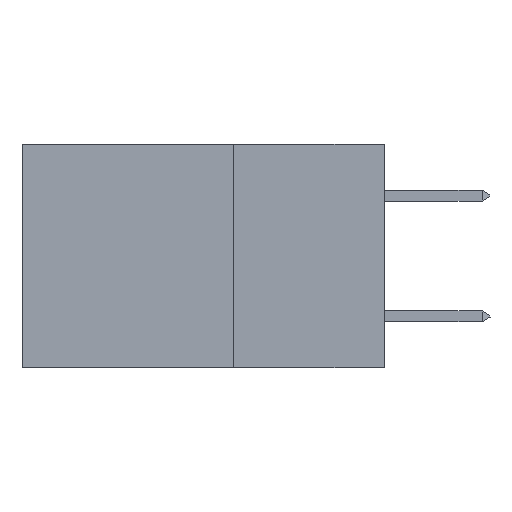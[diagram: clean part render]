
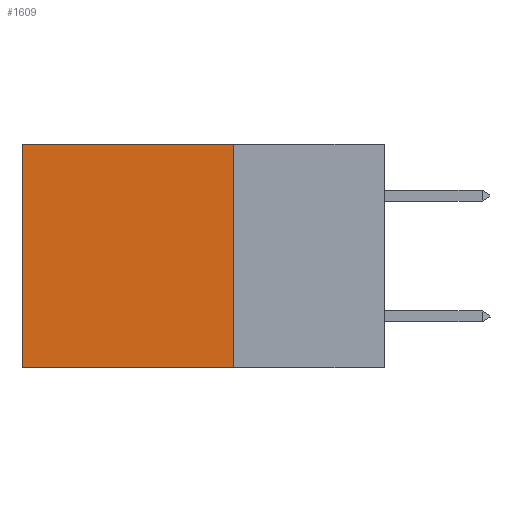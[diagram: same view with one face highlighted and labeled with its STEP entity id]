
A CAD part, left-side view. The second image highlights one B-rep face of the part: STEP entity #1609.
In plain terms, the highlighted planar face has unit normal (-1, 0, 0).
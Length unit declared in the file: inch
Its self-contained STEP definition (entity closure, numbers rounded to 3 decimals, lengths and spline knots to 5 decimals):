
#343 = CARTESIAN_POINT ( 'NONE',  ( 0.2875, 0.25, 0. ) ) ;
#895 = FACE_OUTER_BOUND ( 'NONE', #2288, .T. ) ;
#1002 = CARTESIAN_POINT ( 'NONE',  ( 0.2875, 0.25, -0.37 ) ) ;
#1474 = EDGE_CURVE ( 'NONE', #21234, #15775, #17273, .T. ) ;
#1609 = ADVANCED_FACE ( 'NONE', ( #895 ), #22056, .F. ) ;
#2288 = EDGE_LOOP ( 'NONE', ( #4274, #20066, #19866, #18275 ) ) ;
#3679 = LINE ( 'NONE', #343, #21585 ) ;
#4274 = ORIENTED_EDGE ( 'NONE', *, *, #13010, .T. ) ;
#5453 = CARTESIAN_POINT ( 'NONE',  ( 0.2875, 0.6, -0.37 ) ) ;
#7351 = CARTESIAN_POINT ( 'NONE',  ( 0.2875, 0.6, 0. ) ) ;
#7728 = LINE ( 'NONE', #12226, #21047 ) ;
#8316 = CARTESIAN_POINT ( 'NONE',  ( 0.2875, 0.25, 0. ) ) ;
#8322 = LINE ( 'NONE', #13500, #11852 ) ;
#10091 = DIRECTION ( 'NONE',  ( 0., 1., 0. ) ) ;
#10201 = DIRECTION ( 'NONE',  ( 0., 0., -1. ) ) ;
#10947 = DIRECTION ( 'NONE',  ( 0., 0., -1. ) ) ;
#11852 = VECTOR ( 'NONE', #10091, 39.37008 ) ;
#12226 = CARTESIAN_POINT ( 'NONE',  ( 0.2875, 0.6, 0. ) ) ;
#12547 = EDGE_CURVE ( 'NONE', #21234, #17060, #3679, .T. ) ;
#12642 = VECTOR ( 'NONE', #17256, 39.37008 ) ;
#13010 = EDGE_CURVE ( 'NONE', #15775, #17253, #7728, .T. ) ;
#13500 = CARTESIAN_POINT ( 'NONE',  ( 0.2875, 0.25, -0.37 ) ) ;
#13959 = DIRECTION ( 'NONE',  ( 0., 0., -1. ) ) ;
#15333 = DIRECTION ( 'NONE',  ( 1., 0., 0. ) ) ;
#15775 = VERTEX_POINT ( 'NONE', #7351 ) ;
#16700 = CARTESIAN_POINT ( 'NONE',  ( 0.2875, 0.25, 0. ) ) ;
#16953 = CARTESIAN_POINT ( 'NONE',  ( 0.2875, 0.25, 0. ) ) ;
#17060 = VERTEX_POINT ( 'NONE', #1002 ) ;
#17174 = EDGE_CURVE ( 'NONE', #17060, #17253, #8322, .T. ) ;
#17253 = VERTEX_POINT ( 'NONE', #5453 ) ;
#17256 = DIRECTION ( 'NONE',  ( 0., 1., 0. ) ) ;
#17273 = LINE ( 'NONE', #16700, #12642 ) ;
#18275 = ORIENTED_EDGE ( 'NONE', *, *, #1474, .T. ) ;
#19866 = ORIENTED_EDGE ( 'NONE', *, *, #12547, .F. ) ;
#20066 = ORIENTED_EDGE ( 'NONE', *, *, #17174, .F. ) ;
#21047 = VECTOR ( 'NONE', #13959, 39.37008 ) ;
#21234 = VERTEX_POINT ( 'NONE', #16953 ) ;
#21566 = AXIS2_PLACEMENT_3D ( 'NONE', #8316, #15333, #10201 ) ;
#21585 = VECTOR ( 'NONE', #10947, 39.37008 ) ;
#22056 = PLANE ( 'NONE',  #21566 ) ;
